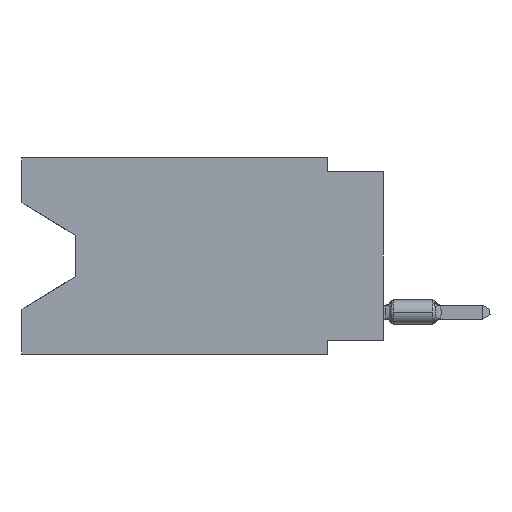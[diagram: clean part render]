
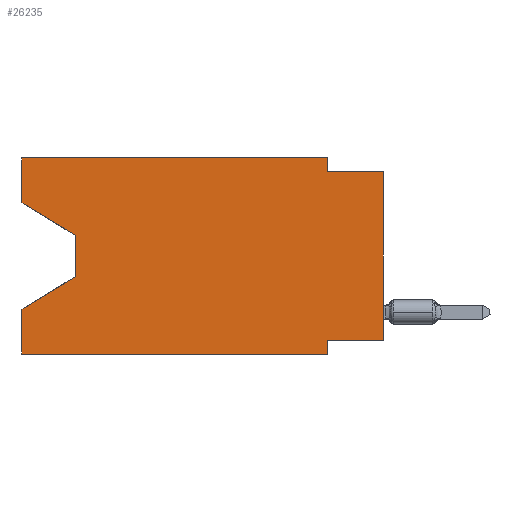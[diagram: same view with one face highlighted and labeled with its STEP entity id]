
A CAD part, left-side view. The second image highlights one B-rep face of the part: STEP entity #26235.
In plain terms, the highlighted planar face has unit normal (-1, 0, 0).
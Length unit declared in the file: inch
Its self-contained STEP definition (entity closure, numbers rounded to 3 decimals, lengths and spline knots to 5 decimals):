
#1377 = EDGE_CURVE ( 'NONE', #35653, #15796, #23378, .T. ) ;
#1585 = CARTESIAN_POINT ( 'NONE',  ( 0., 0.1, 0. ) ) ;
#1794 = EDGE_CURVE ( 'NONE', #5354, #1976, #28593, .T. ) ;
#1976 = VERTEX_POINT ( 'NONE', #30691 ) ;
#2031 = EDGE_CURVE ( 'NONE', #17186, #1976, #30295, .T. ) ;
#2178 = EDGE_CURVE ( 'NONE', #19660, #34751, #16730, .T. ) ;
#2257 = ORIENTED_EDGE ( 'NONE', *, *, #8721, .T. ) ;
#2325 = CARTESIAN_POINT ( 'NONE',  ( 0., 0.1, -0.025 ) ) ;
#2450 = EDGE_LOOP ( 'NONE', ( #2257, #26227, #34613, #7857, #35868, #30225, #35760, #32464, #37016, #11274, #5784, #31215 ) ) ;
#2971 = DIRECTION ( 'NONE',  ( 0., -1., 0. ) ) ;
#3343 = CARTESIAN_POINT ( 'NONE',  ( 0., 0., -0.025 ) ) ;
#3451 = CARTESIAN_POINT ( 'NONE',  ( 0., 0.55, -0.138 ) ) ;
#4023 = LINE ( 'NONE', #3451, #13088 ) ;
#4108 = LINE ( 'NONE', #1585, #35688 ) ;
#4350 = VERTEX_POINT ( 'NONE', #31253 ) ;
#5231 = DIRECTION ( 'NONE',  ( 0., 1., 0. ) ) ;
#5251 = EDGE_CURVE ( 'NONE', #35653, #34751, #35271, .T. ) ;
#5354 = VERTEX_POINT ( 'NONE', #30624 ) ;
#5592 = VECTOR ( 'NONE', #14217, 39.37008 ) ;
#5742 = VECTOR ( 'NONE', #38024, 39.37008 ) ;
#5784 = ORIENTED_EDGE ( 'NONE', *, *, #8383, .F. ) ;
#5869 = CARTESIAN_POINT ( 'NONE',  ( 0., 0.645, 0. ) ) ;
#7857 = ORIENTED_EDGE ( 'NONE', *, *, #1794, .F. ) ;
#7919 = CARTESIAN_POINT ( 'NONE',  ( 0., 0., -0.325 ) ) ;
#8139 = AXIS2_PLACEMENT_3D ( 'NONE', #27152, #22101, #36040 ) ;
#8311 = CARTESIAN_POINT ( 'NONE',  ( 0., 0., -0.325 ) ) ;
#8383 = EDGE_CURVE ( 'NONE', #4350, #14077, #20573, .T. ) ;
#8440 = VERTEX_POINT ( 'NONE', #24980 ) ;
#8525 = CARTESIAN_POINT ( 'NONE',  ( 0., 0.1, -0.325 ) ) ;
#8566 = LINE ( 'NONE', #20181, #18214 ) ;
#8706 = CARTESIAN_POINT ( 'NONE',  ( 0., 0.645, -0.08025 ) ) ;
#8721 = EDGE_CURVE ( 'NONE', #9175, #20112, #20708, .T. ) ;
#9059 = CARTESIAN_POINT ( 'NONE',  ( 0., 0.645, -0.08025 ) ) ;
#9175 = VERTEX_POINT ( 'NONE', #9059 ) ;
#9191 = EDGE_CURVE ( 'NONE', #20112, #17186, #4023, .T. ) ;
#10297 = CARTESIAN_POINT ( 'NONE',  ( 0., 0., 0. ) ) ;
#10908 = CARTESIAN_POINT ( 'NONE',  ( 0., 0.55, -0.138 ) ) ;
#11274 = ORIENTED_EDGE ( 'NONE', *, *, #15645, .F. ) ;
#13088 = VECTOR ( 'NONE', #21034, 39.37008 ) ;
#14077 = VERTEX_POINT ( 'NONE', #17643 ) ;
#14217 = DIRECTION ( 'NONE',  ( 0., 0., -1. ) ) ;
#15645 = EDGE_CURVE ( 'NONE', #14077, #19660, #4108, .T. ) ;
#15796 = VERTEX_POINT ( 'NONE', #8525 ) ;
#15891 = DIRECTION ( 'NONE',  ( 0., 0., -1. ) ) ;
#15918 = PLANE ( 'NONE',  #8139 ) ;
#15973 = DIRECTION ( 'NONE',  ( 0., 0.855, -0.519 ) ) ;
#16057 = VECTOR ( 'NONE', #15973, 39.37008 ) ;
#16730 = LINE ( 'NONE', #28546, #5742 ) ;
#17186 = VERTEX_POINT ( 'NONE', #25431 ) ;
#17643 = CARTESIAN_POINT ( 'NONE',  ( 0., 0.1, 0. ) ) ;
#18000 = VECTOR ( 'NONE', #5231, 39.37008 ) ;
#18214 = VECTOR ( 'NONE', #20360, 39.37008 ) ;
#18498 = VECTOR ( 'NONE', #25872, 39.37008 ) ;
#18611 = FACE_OUTER_BOUND ( 'NONE', #2450, .T. ) ;
#18996 = DIRECTION ( 'NONE',  ( 0., 0., 1. ) ) ;
#19660 = VERTEX_POINT ( 'NONE', #2325 ) ;
#20076 = EDGE_CURVE ( 'NONE', #5354, #8440, #24838, .T. ) ;
#20112 = VERTEX_POINT ( 'NONE', #10908 ) ;
#20181 = CARTESIAN_POINT ( 'NONE',  ( 0., 0.645, 0. ) ) ;
#20360 = DIRECTION ( 'NONE',  ( 0., 0., 1. ) ) ;
#20573 = LINE ( 'NONE', #5869, #33443 ) ;
#20708 = LINE ( 'NONE', #8706, #21099 ) ;
#21034 = DIRECTION ( 'NONE',  ( 0., 0., -1. ) ) ;
#21099 = VECTOR ( 'NONE', #35768, 39.37008 ) ;
#22101 = DIRECTION ( 'NONE',  ( 1., 0., 0. ) ) ;
#22346 = CARTESIAN_POINT ( 'NONE',  ( 0., 0.1, -0.35 ) ) ;
#22578 = CARTESIAN_POINT ( 'NONE',  ( 0., 0.645, 0. ) ) ;
#23378 = LINE ( 'NONE', #7919, #18000 ) ;
#24838 = LINE ( 'NONE', #36655, #37868 ) ;
#24980 = CARTESIAN_POINT ( 'NONE',  ( 0., 0.1, -0.35 ) ) ;
#25252 = CARTESIAN_POINT ( 'NONE',  ( 0., 0.55, -0.212 ) ) ;
#25431 = CARTESIAN_POINT ( 'NONE',  ( 0., 0.55, -0.212 ) ) ;
#25872 = DIRECTION ( 'NONE',  ( 0., 0., 1. ) ) ;
#26227 = ORIENTED_EDGE ( 'NONE', *, *, #9191, .T. ) ;
#26235 = ADVANCED_FACE ( 'NONE', ( #18611 ), #15918, .F. ) ;
#27152 = CARTESIAN_POINT ( 'NONE',  ( 0., 0.645, 0. ) ) ;
#28546 = CARTESIAN_POINT ( 'NONE',  ( 0., 0., -0.025 ) ) ;
#28593 = LINE ( 'NONE', #22578, #18498 ) ;
#29640 = VECTOR ( 'NONE', #18996, 39.37008 ) ;
#30225 = ORIENTED_EDGE ( 'NONE', *, *, #37691, .F. ) ;
#30268 = DIRECTION ( 'NONE',  ( 0., -1., 0. ) ) ;
#30295 = LINE ( 'NONE', #25252, #16057 ) ;
#30624 = CARTESIAN_POINT ( 'NONE',  ( 0., 0.645, -0.35 ) ) ;
#30691 = CARTESIAN_POINT ( 'NONE',  ( 0., 0.645, -0.26975 ) ) ;
#31215 = ORIENTED_EDGE ( 'NONE', *, *, #38259, .F. ) ;
#31253 = CARTESIAN_POINT ( 'NONE',  ( 0., 0.645, 0. ) ) ;
#32464 = ORIENTED_EDGE ( 'NONE', *, *, #5251, .T. ) ;
#33443 = VECTOR ( 'NONE', #2971, 39.37008 ) ;
#34613 = ORIENTED_EDGE ( 'NONE', *, *, #2031, .T. ) ;
#34751 = VERTEX_POINT ( 'NONE', #3343 ) ;
#35271 = LINE ( 'NONE', #10297, #29640 ) ;
#35653 = VERTEX_POINT ( 'NONE', #8311 ) ;
#35688 = VECTOR ( 'NONE', #15891, 39.37008 ) ;
#35760 = ORIENTED_EDGE ( 'NONE', *, *, #1377, .F. ) ;
#35768 = DIRECTION ( 'NONE',  ( 0., -0.855, -0.519 ) ) ;
#35868 = ORIENTED_EDGE ( 'NONE', *, *, #20076, .T. ) ;
#36040 = DIRECTION ( 'NONE',  ( 0., 0., -1. ) ) ;
#36655 = CARTESIAN_POINT ( 'NONE',  ( 0., 0.645, -0.35 ) ) ;
#37016 = ORIENTED_EDGE ( 'NONE', *, *, #2178, .F. ) ;
#37057 = LINE ( 'NONE', #22346, #5592 ) ;
#37691 = EDGE_CURVE ( 'NONE', #15796, #8440, #37057, .T. ) ;
#37868 = VECTOR ( 'NONE', #30268, 39.37008 ) ;
#38024 = DIRECTION ( 'NONE',  ( 0., -1., 0. ) ) ;
#38259 = EDGE_CURVE ( 'NONE', #9175, #4350, #8566, .T. ) ;
